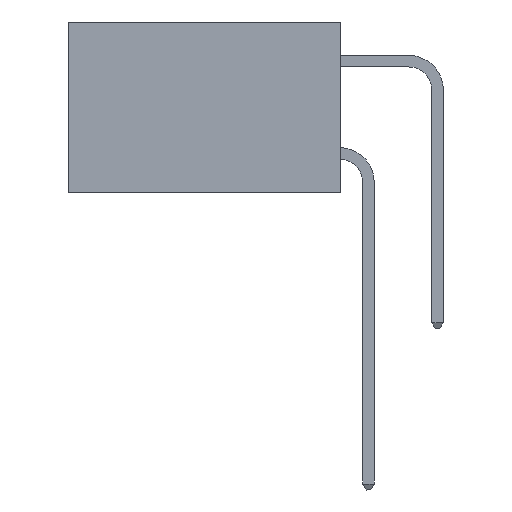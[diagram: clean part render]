
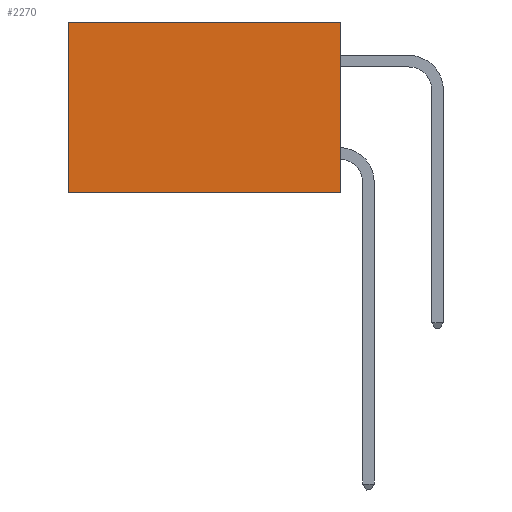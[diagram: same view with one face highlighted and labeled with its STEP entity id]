
A CAD part, left-side view. The second image highlights one B-rep face of the part: STEP entity #2270.
In plain terms, the highlighted planar face has unit normal (-1, 0, 0).
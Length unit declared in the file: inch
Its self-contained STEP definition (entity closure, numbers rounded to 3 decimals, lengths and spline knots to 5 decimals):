
#186 = DIRECTION ( 'NONE',  ( 0., 0., -1. ) ) ;
#207 = DIRECTION ( 'NONE',  ( 1., 0., 0. ) ) ;
#228 = CARTESIAN_POINT ( 'NONE',  ( 0.277, 0., -0.37 ) ) ;
#445 = PLANE ( 'NONE',  #15932 ) ;
#611 = ORIENTED_EDGE ( 'NONE', *, *, #8669, .F. ) ;
#679 = CARTESIAN_POINT ( 'NONE',  ( 0.277, 0., -0.37 ) ) ;
#750 = DIRECTION ( 'NONE',  ( 0., 1., 0. ) ) ;
#1304 = EDGE_CURVE ( 'NONE', #11833, #1757, #6559, .T. ) ;
#1757 = VERTEX_POINT ( 'NONE', #10861 ) ;
#2270 = ADVANCED_FACE ( 'NONE', ( #12445 ), #445, .F. ) ;
#3416 = CARTESIAN_POINT ( 'NONE',  ( 0.277, 0.59, -0.37 ) ) ;
#3961 = ORIENTED_EDGE ( 'NONE', *, *, #10109, .T. ) ;
#4772 = VECTOR ( 'NONE', #7167, 39.37008 ) ;
#5810 = CARTESIAN_POINT ( 'NONE',  ( 0.277, 0., 0. ) ) ;
#6094 = VERTEX_POINT ( 'NONE', #10015 ) ;
#6559 = LINE ( 'NONE', #9725, #10158 ) ;
#6714 = LINE ( 'NONE', #679, #9894 ) ;
#7167 = DIRECTION ( 'NONE',  ( 0., 1., 0. ) ) ;
#7377 = DIRECTION ( 'NONE',  ( 0., 0., -1. ) ) ;
#8669 = EDGE_CURVE ( 'NONE', #6094, #11833, #6714, .T. ) ;
#8779 = LINE ( 'NONE', #5810, #4772 ) ;
#8976 = VECTOR ( 'NONE', #14183, 39.37008 ) ;
#9725 = CARTESIAN_POINT ( 'NONE',  ( 0.277, 0., -0.37 ) ) ;
#9894 = VECTOR ( 'NONE', #7377, 39.37008 ) ;
#9927 = EDGE_CURVE ( 'NONE', #6094, #14632, #8779, .T. ) ;
#10015 = CARTESIAN_POINT ( 'NONE',  ( 0.277, 0., 0. ) ) ;
#10109 = EDGE_CURVE ( 'NONE', #14632, #1757, #12591, .T. ) ;
#10127 = CARTESIAN_POINT ( 'NONE',  ( 0.277, 0.59, 0. ) ) ;
#10158 = VECTOR ( 'NONE', #750, 39.37008 ) ;
#10425 = EDGE_LOOP ( 'NONE', ( #3961, #15916, #611, #14453 ) ) ;
#10861 = CARTESIAN_POINT ( 'NONE',  ( 0.277, 0.59, -0.37 ) ) ;
#11833 = VERTEX_POINT ( 'NONE', #14003 ) ;
#12445 = FACE_OUTER_BOUND ( 'NONE', #10425, .T. ) ;
#12591 = LINE ( 'NONE', #3416, #8976 ) ;
#14003 = CARTESIAN_POINT ( 'NONE',  ( 0.277, 0., -0.37 ) ) ;
#14183 = DIRECTION ( 'NONE',  ( 0., 0., -1. ) ) ;
#14453 = ORIENTED_EDGE ( 'NONE', *, *, #9927, .T. ) ;
#14632 = VERTEX_POINT ( 'NONE', #10127 ) ;
#15916 = ORIENTED_EDGE ( 'NONE', *, *, #1304, .F. ) ;
#15932 = AXIS2_PLACEMENT_3D ( 'NONE', #228, #207, #186 ) ;
